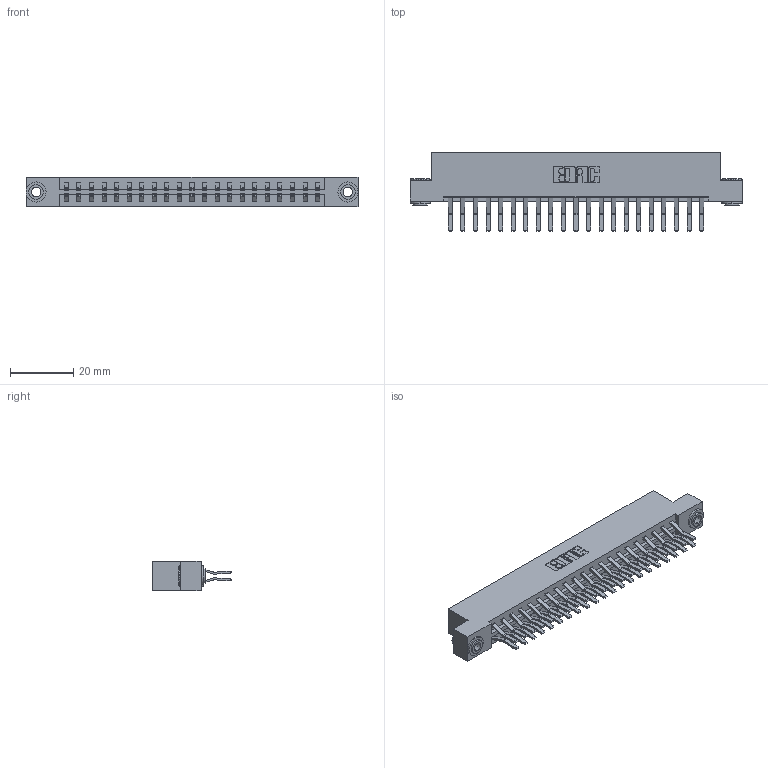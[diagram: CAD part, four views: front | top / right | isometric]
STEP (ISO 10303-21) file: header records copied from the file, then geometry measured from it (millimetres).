
FILE_DESCRIPTION (( 'STEP AP203' ), '1' );
FILE_NAME ('833-042-560-203.STEP', '2020-06-03T22:57:43', ( '' ), ( '' ), 'SwSTEP 2.0', 'SolidWorks 2020', '' );
FILE_SCHEMA (( 'CONFIG_CONTROL_DESIGN' ));
Length unit declared in the file: inch
Products named in the file (4): 345-250-002_345-250-002-102; 833-042-560-203; 345-292-001_560 Tail; 833 Part_Flush - .156 Dia - TH
Assembly tree (45 placements, depth 2):
  833-042-560-203
    833 Part_Flush - .156 Dia - TH
    345-292-001_560 Tail  x42
    345-250-002_345-250-002-102  x2
Bounding box: 104.75 x 24.78 x 9.4 mm (x, y, z)
Volume: 10792.6 mm3; surface area: 13540.1 mm2
Topology: 45 solids, 45 shells, 2420 faces, 7149 edges, 4706 vertices
Faces by surface type: plane 1592, cylinder 820, cone 8
Entity records: 16964 total; most frequent: CARTESIAN_POINT 2813, ORIENTED_EDGE 2742, DIRECTION 2477, EDGE_CURVE 1371, LINE 1215, VECTOR 1215, VERTEX_POINT 910, AXIS2_PLACEMENT_3D 631
